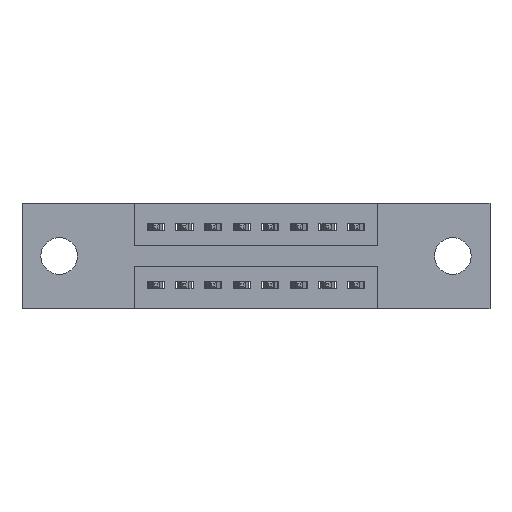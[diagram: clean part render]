
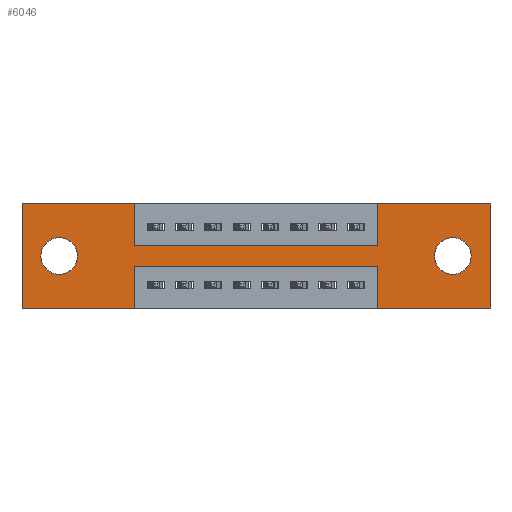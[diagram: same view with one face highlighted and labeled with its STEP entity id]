
A CAD part, front view. The second image highlights one B-rep face of the part: STEP entity #6046.
In plain terms, the highlighted planar face has unit normal (0, -1, 0).
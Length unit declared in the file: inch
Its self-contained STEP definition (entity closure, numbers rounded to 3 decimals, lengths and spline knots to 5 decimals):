
#19 = EDGE_CURVE ( 'NONE', #10133, #2826, #10437, .T. ) ;
#139 = VECTOR ( 'NONE', #2193, 39.37008 ) ;
#188 = EDGE_CURVE ( 'NONE', #1682, #9045, #3103, .T. ) ;
#335 = VECTOR ( 'NONE', #4487, 39.37008 ) ;
#454 = CARTESIAN_POINT ( 'NONE',  ( 1.2425, 0., 0. ) ) ;
#579 = CIRCLE ( 'NONE', #3385, 0.064 ) ;
#589 = CARTESIAN_POINT ( 'NONE',  ( 1.505, 0., -0.185 ) ) ;
#604 = VERTEX_POINT ( 'NONE', #3861 ) ;
#647 = CARTESIAN_POINT ( 'NONE',  ( 0., 0., 0. ) ) ;
#682 = VECTOR ( 'NONE', #8262, 39.37008 ) ;
#946 = CARTESIAN_POINT ( 'NONE',  ( 0., 0., 0. ) ) ;
#985 = CARTESIAN_POINT ( 'NONE',  ( 0., 0., 0. ) ) ;
#986 = AXIS2_PLACEMENT_3D ( 'NONE', #589, #5803, #7699 ) ;
#1085 = ORIENTED_EDGE ( 'NONE', *, *, #4044, .F. ) ;
#1192 = CARTESIAN_POINT ( 'NONE',  ( 1.505, 0., -0.249 ) ) ;
#1228 = DIRECTION ( 'NONE',  ( 0., 0., 1. ) ) ;
#1294 = ORIENTED_EDGE ( 'NONE', *, *, #3898, .F. ) ;
#1327 = LINE ( 'NONE', #7828, #3984 ) ;
#1457 = CIRCLE ( 'NONE', #3534, 0.064 ) ;
#1479 = ORIENTED_EDGE ( 'NONE', *, *, #10674, .T. ) ;
#1500 = VECTOR ( 'NONE', #5019, 39.37008 ) ;
#1569 = DIRECTION ( 'NONE',  ( 0., 1., 0. ) ) ;
#1661 = VECTOR ( 'NONE', #7078, 39.37008 ) ;
#1682 = VERTEX_POINT ( 'NONE', #10286 ) ;
#1750 = CARTESIAN_POINT ( 'NONE',  ( 1.2425, 0., 0. ) ) ;
#1774 = DIRECTION ( 'NONE',  ( 0., 0., 1. ) ) ;
#1781 = CARTESIAN_POINT ( 'NONE',  ( 1.635, 0., -0.37 ) ) ;
#1836 = CARTESIAN_POINT ( 'NONE',  ( 1.505, 0., -0.121 ) ) ;
#2003 = CARTESIAN_POINT ( 'NONE',  ( 0., 0., -0.37 ) ) ;
#2193 = DIRECTION ( 'NONE',  ( -1., 0., 0. ) ) ;
#2244 = FACE_BOUND ( 'NONE', #3306, .T. ) ;
#2333 = AXIS2_PLACEMENT_3D ( 'NONE', #6187, #9641, #1228 ) ;
#2405 = CARTESIAN_POINT ( 'NONE',  ( 1.2425, 0., -0.37 ) ) ;
#2487 = EDGE_CURVE ( 'NONE', #7343, #4309, #2911, .T. ) ;
#2588 = CARTESIAN_POINT ( 'NONE',  ( 0.3925, 0., -0.15 ) ) ;
#2686 = ORIENTED_EDGE ( 'NONE', *, *, #188, .F. ) ;
#2826 = VERTEX_POINT ( 'NONE', #1781 ) ;
#2911 = CIRCLE ( 'NONE', #2333, 0.064 ) ;
#2934 = DIRECTION ( 'NONE',  ( 1., 0., 0. ) ) ;
#3030 = ORIENTED_EDGE ( 'NONE', *, *, #7346, .F. ) ;
#3103 = LINE ( 'NONE', #2405, #682 ) ;
#3189 = EDGE_CURVE ( 'NONE', #8157, #6813, #6018, .T. ) ;
#3210 = ORIENTED_EDGE ( 'NONE', *, *, #6492, .F. ) ;
#3224 = AXIS2_PLACEMENT_3D ( 'NONE', #5493, #3795, #10464 ) ;
#3257 = EDGE_CURVE ( 'NONE', #9611, #10149, #7218, .T. ) ;
#3306 = EDGE_LOOP ( 'NONE', ( #9947, #1479 ) ) ;
#3319 = ORIENTED_EDGE ( 'NONE', *, *, #3189, .F. ) ;
#3343 = VECTOR ( 'NONE', #3479, 39.37008 ) ;
#3385 = AXIS2_PLACEMENT_3D ( 'NONE', #10749, #1569, #7457 ) ;
#3479 = DIRECTION ( 'NONE',  ( 0., 0., -1. ) ) ;
#3534 = AXIS2_PLACEMENT_3D ( 'NONE', #6547, #5109, #1774 ) ;
#3615 = CARTESIAN_POINT ( 'NONE',  ( 1.635, 0., 0. ) ) ;
#3657 = LINE ( 'NONE', #10555, #1661 ) ;
#3686 = LINE ( 'NONE', #946, #5758 ) ;
#3709 = ORIENTED_EDGE ( 'NONE', *, *, #9026, .F. ) ;
#3730 = PLANE ( 'NONE',  #3224 ) ;
#3753 = ORIENTED_EDGE ( 'NONE', *, *, #3257, .T. ) ;
#3764 = CARTESIAN_POINT ( 'NONE',  ( 0.3925, 0., -0.37 ) ) ;
#3773 = LINE ( 'NONE', #4530, #335 ) ;
#3795 = DIRECTION ( 'NONE',  ( 0., -1., 0. ) ) ;
#3861 = CARTESIAN_POINT ( 'NONE',  ( 1.2425, 0., -0.15 ) ) ;
#3864 = CARTESIAN_POINT ( 'NONE',  ( 0.3925, 0., -0.15 ) ) ;
#3898 = EDGE_CURVE ( 'NONE', #7945, #9985, #9225, .T. ) ;
#3934 = FACE_OUTER_BOUND ( 'NONE', #5976, .T. ) ;
#3984 = VECTOR ( 'NONE', #7793, 39.37008 ) ;
#4044 = EDGE_CURVE ( 'NONE', #9045, #10444, #1327, .T. ) ;
#4075 = CARTESIAN_POINT ( 'NONE',  ( 0.3925, 0., -0.22 ) ) ;
#4309 = VERTEX_POINT ( 'NONE', #5528 ) ;
#4357 = LINE ( 'NONE', #5552, #139 ) ;
#4391 = CARTESIAN_POINT ( 'NONE',  ( 1.2425, 0., -0.22 ) ) ;
#4476 = CARTESIAN_POINT ( 'NONE',  ( 1.635, 0., 0. ) ) ;
#4487 = DIRECTION ( 'NONE',  ( -1., 0., 0. ) ) ;
#4530 = CARTESIAN_POINT ( 'NONE',  ( 0., 0., -0.37 ) ) ;
#4538 = EDGE_CURVE ( 'NONE', #2826, #1682, #4357, .T. ) ;
#4789 = EDGE_LOOP ( 'NONE', ( #3753, #8888 ) ) ;
#4885 = VECTOR ( 'NONE', #8146, 39.37008 ) ;
#4939 = CARTESIAN_POINT ( 'NONE',  ( 0.3925, 0., 0. ) ) ;
#5019 = DIRECTION ( 'NONE',  ( 0., 0., 1. ) ) ;
#5053 = VECTOR ( 'NONE', #8560, 39.37008 ) ;
#5109 = DIRECTION ( 'NONE',  ( 0., 1., 0. ) ) ;
#5411 = EDGE_CURVE ( 'NONE', #7279, #10133, #3686, .T. ) ;
#5464 = CARTESIAN_POINT ( 'NONE',  ( 0.13, 0., -0.121 ) ) ;
#5493 = CARTESIAN_POINT ( 'NONE',  ( 0., 0., -0.37 ) ) ;
#5528 = CARTESIAN_POINT ( 'NONE',  ( 0.13, 0., -0.249 ) ) ;
#5551 = VERTEX_POINT ( 'NONE', #3764 ) ;
#5552 = CARTESIAN_POINT ( 'NONE',  ( 0., 0., -0.37 ) ) ;
#5758 = VECTOR ( 'NONE', #6847, 39.37008 ) ;
#5803 = DIRECTION ( 'NONE',  ( 0., 1., 0. ) ) ;
#5976 = EDGE_LOOP ( 'NONE', ( #3030, #1085, #2686, #9283, #6671, #7307, #3709, #6270, #1294, #3210, #3319, #9509 ) ) ;
#6018 = LINE ( 'NONE', #647, #8006 ) ;
#6021 = LINE ( 'NONE', #8820, #8662 ) ;
#6046 = ADVANCED_FACE ( 'NONE', ( #8409, #2244, #3934 ), #3730, .T. ) ;
#6187 = CARTESIAN_POINT ( 'NONE',  ( 0.13, 0., -0.185 ) ) ;
#6270 = ORIENTED_EDGE ( 'NONE', *, *, #10333, .F. ) ;
#6492 = EDGE_CURVE ( 'NONE', #6813, #7945, #6021, .T. ) ;
#6547 = CARTESIAN_POINT ( 'NONE',  ( 0.13, 0., -0.185 ) ) ;
#6625 = LINE ( 'NONE', #1750, #1500 ) ;
#6671 = ORIENTED_EDGE ( 'NONE', *, *, #19, .F. ) ;
#6813 = VERTEX_POINT ( 'NONE', #985 ) ;
#6847 = DIRECTION ( 'NONE',  ( 1., 0., 0. ) ) ;
#7078 = DIRECTION ( 'NONE',  ( 0., 0., -1. ) ) ;
#7218 = CIRCLE ( 'NONE', #986, 0.064 ) ;
#7279 = VERTEX_POINT ( 'NONE', #454 ) ;
#7307 = ORIENTED_EDGE ( 'NONE', *, *, #5411, .F. ) ;
#7343 = VERTEX_POINT ( 'NONE', #5464 ) ;
#7346 = EDGE_CURVE ( 'NONE', #10444, #5551, #3657, .T. ) ;
#7457 = DIRECTION ( 'NONE',  ( 0., 0., -1. ) ) ;
#7699 = DIRECTION ( 'NONE',  ( 0., 0., -1. ) ) ;
#7793 = DIRECTION ( 'NONE',  ( -1., 0., 0. ) ) ;
#7828 = CARTESIAN_POINT ( 'NONE',  ( 0.3925, 0., -0.22 ) ) ;
#7945 = VERTEX_POINT ( 'NONE', #4939 ) ;
#8006 = VECTOR ( 'NONE', #10659, 39.37008 ) ;
#8146 = DIRECTION ( 'NONE',  ( 1., 0., 0. ) ) ;
#8157 = VERTEX_POINT ( 'NONE', #2003 ) ;
#8188 = EDGE_CURVE ( 'NONE', #5551, #8157, #3773, .T. ) ;
#8262 = DIRECTION ( 'NONE',  ( 0., 0., 1. ) ) ;
#8341 = EDGE_CURVE ( 'NONE', #10149, #9611, #579, .T. ) ;
#8409 = FACE_BOUND ( 'NONE', #4789, .T. ) ;
#8560 = DIRECTION ( 'NONE',  ( 0., 0., -1. ) ) ;
#8662 = VECTOR ( 'NONE', #2934, 39.37008 ) ;
#8820 = CARTESIAN_POINT ( 'NONE',  ( 0., 0., 0. ) ) ;
#8888 = ORIENTED_EDGE ( 'NONE', *, *, #8341, .T. ) ;
#9026 = EDGE_CURVE ( 'NONE', #604, #7279, #6625, .T. ) ;
#9045 = VERTEX_POINT ( 'NONE', #4391 ) ;
#9225 = LINE ( 'NONE', #10865, #3343 ) ;
#9283 = ORIENTED_EDGE ( 'NONE', *, *, #4538, .F. ) ;
#9509 = ORIENTED_EDGE ( 'NONE', *, *, #8188, .F. ) ;
#9611 = VERTEX_POINT ( 'NONE', #1836 ) ;
#9641 = DIRECTION ( 'NONE',  ( 0., 1., 0. ) ) ;
#9947 = ORIENTED_EDGE ( 'NONE', *, *, #2487, .T. ) ;
#9985 = VERTEX_POINT ( 'NONE', #2588 ) ;
#10133 = VERTEX_POINT ( 'NONE', #3615 ) ;
#10149 = VERTEX_POINT ( 'NONE', #1192 ) ;
#10286 = CARTESIAN_POINT ( 'NONE',  ( 1.2425, 0., -0.37 ) ) ;
#10333 = EDGE_CURVE ( 'NONE', #9985, #604, #10675, .T. ) ;
#10437 = LINE ( 'NONE', #4476, #5053 ) ;
#10444 = VERTEX_POINT ( 'NONE', #4075 ) ;
#10464 = DIRECTION ( 'NONE',  ( 0., 0., -1. ) ) ;
#10555 = CARTESIAN_POINT ( 'NONE',  ( 0.3925, 0., -0.37 ) ) ;
#10659 = DIRECTION ( 'NONE',  ( 0., 0., 1. ) ) ;
#10674 = EDGE_CURVE ( 'NONE', #4309, #7343, #1457, .T. ) ;
#10675 = LINE ( 'NONE', #3864, #4885 ) ;
#10749 = CARTESIAN_POINT ( 'NONE',  ( 1.505, 0., -0.185 ) ) ;
#10865 = CARTESIAN_POINT ( 'NONE',  ( 0.3925, 0., 0. ) ) ;
